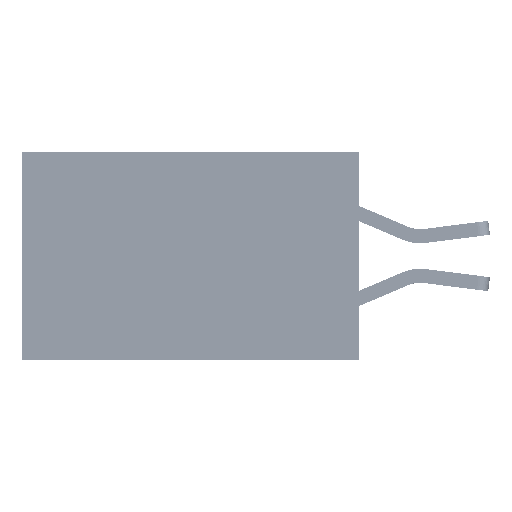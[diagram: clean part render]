
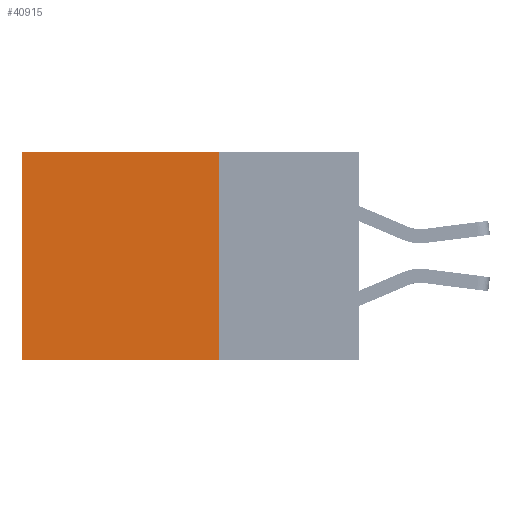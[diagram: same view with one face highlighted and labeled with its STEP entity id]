
A CAD part, left-side view. The second image highlights one B-rep face of the part: STEP entity #40915.
In plain terms, the highlighted planar face has unit normal (-1, 0, 0).
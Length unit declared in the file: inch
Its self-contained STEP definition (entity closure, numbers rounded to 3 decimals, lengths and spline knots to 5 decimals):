
#828 = DIRECTION ( 'NONE',  ( 1., 0., 0. ) ) ;
#866 = ORIENTED_EDGE ( 'NONE', *, *, #24595, .F. ) ;
#1123 = CARTESIAN_POINT ( 'NONE',  ( 0.2875, 0.6, -0.37 ) ) ;
#1261 = VECTOR ( 'NONE', #34220, 39.37008 ) ;
#2035 = CARTESIAN_POINT ( 'NONE',  ( 0.2875, 0.6, 0. ) ) ;
#3082 = EDGE_CURVE ( 'NONE', #4109, #30107, #30808, .T. ) ;
#3420 = LINE ( 'NONE', #13927, #48168 ) ;
#4109 = VERTEX_POINT ( 'NONE', #2035 ) ;
#8925 = DIRECTION ( 'NONE',  ( 0., 0., -1. ) ) ;
#9679 = LINE ( 'NONE', #37873, #12208 ) ;
#11967 = LINE ( 'NONE', #42148, #1261 ) ;
#12208 = VECTOR ( 'NONE', #29409, 39.37008 ) ;
#12406 = AXIS2_PLACEMENT_3D ( 'NONE', #49083, #828, #8925 ) ;
#13139 = PLANE ( 'NONE',  #12406 ) ;
#13927 = CARTESIAN_POINT ( 'NONE',  ( 0.2875, 0.25, 0. ) ) ;
#14713 = CARTESIAN_POINT ( 'NONE',  ( 0.2875, 0.6, 0. ) ) ;
#18349 = VERTEX_POINT ( 'NONE', #34755 ) ;
#19446 = EDGE_CURVE ( 'NONE', #24057, #4109, #11967, .T. ) ;
#20506 = EDGE_LOOP ( 'NONE', ( #42413, #866, #32430, #49212 ) ) ;
#21979 = VECTOR ( 'NONE', #30747, 39.37008 ) ;
#24057 = VERTEX_POINT ( 'NONE', #28078 ) ;
#24595 = EDGE_CURVE ( 'NONE', #18349, #30107, #9679, .T. ) ;
#25560 = DIRECTION ( 'NONE',  ( 0., 0., -1. ) ) ;
#26366 = FACE_OUTER_BOUND ( 'NONE', #20506, .T. ) ;
#28078 = CARTESIAN_POINT ( 'NONE',  ( 0.2875, 0.25, 0. ) ) ;
#29409 = DIRECTION ( 'NONE',  ( 0., 1., 0. ) ) ;
#30107 = VERTEX_POINT ( 'NONE', #1123 ) ;
#30747 = DIRECTION ( 'NONE',  ( 0., 0., -1. ) ) ;
#30808 = LINE ( 'NONE', #14713, #21979 ) ;
#32430 = ORIENTED_EDGE ( 'NONE', *, *, #40154, .F. ) ;
#34220 = DIRECTION ( 'NONE',  ( 0., 1., 0. ) ) ;
#34755 = CARTESIAN_POINT ( 'NONE',  ( 0.2875, 0.25, -0.37 ) ) ;
#37873 = CARTESIAN_POINT ( 'NONE',  ( 0.2875, 0.25, -0.37 ) ) ;
#40154 = EDGE_CURVE ( 'NONE', #24057, #18349, #3420, .T. ) ;
#40915 = ADVANCED_FACE ( 'NONE', ( #26366 ), #13139, .F. ) ;
#42148 = CARTESIAN_POINT ( 'NONE',  ( 0.2875, 0.25, 0. ) ) ;
#42413 = ORIENTED_EDGE ( 'NONE', *, *, #3082, .T. ) ;
#48168 = VECTOR ( 'NONE', #25560, 39.37008 ) ;
#49083 = CARTESIAN_POINT ( 'NONE',  ( 0.2875, 0.25, 0. ) ) ;
#49212 = ORIENTED_EDGE ( 'NONE', *, *, #19446, .T. ) ;
